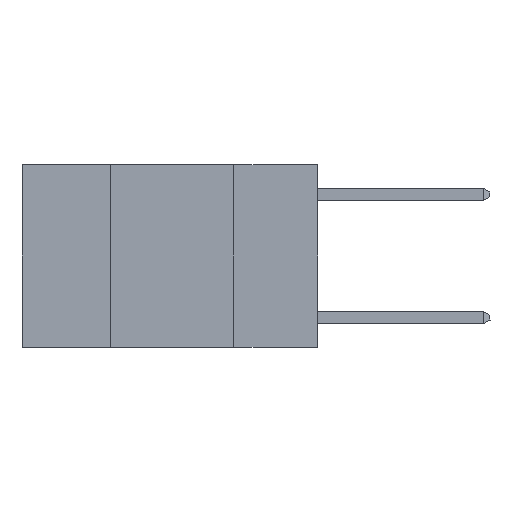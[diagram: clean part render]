
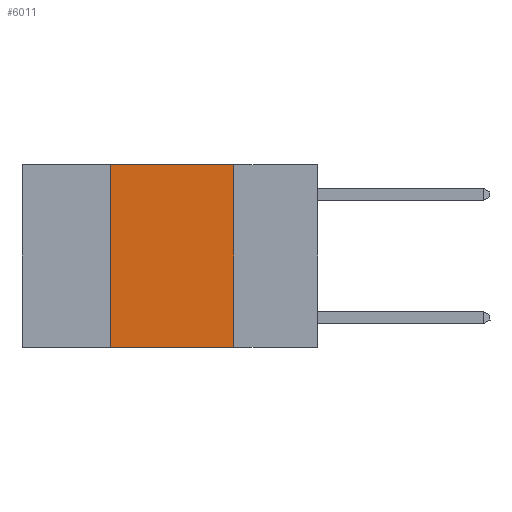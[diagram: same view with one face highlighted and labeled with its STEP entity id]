
A CAD part, left-side view. The second image highlights one B-rep face of the part: STEP entity #6011.
In plain terms, the highlighted planar face has unit normal (-1, 0, 0).
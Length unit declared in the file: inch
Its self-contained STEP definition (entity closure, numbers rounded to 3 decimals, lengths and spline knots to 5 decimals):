
#109 = DIRECTION ( 'NONE',  ( 0., 0., 1. ) ) ;
#329 = PLANE ( 'NONE',  #5812 ) ;
#442 = EDGE_CURVE ( 'NONE', #3343, #728, #18979, .T. ) ;
#728 = VERTEX_POINT ( 'NONE', #13109 ) ;
#1033 = FACE_OUTER_BOUND ( 'NONE', #8221, .T. ) ;
#1705 = ORIENTED_EDGE ( 'NONE', *, *, #16917, .F. ) ;
#2142 = DIRECTION ( 'NONE',  ( 0., 0., -1. ) ) ;
#2422 = VECTOR ( 'NONE', #9090, 39.37008 ) ;
#2716 = DIRECTION ( 'NONE',  ( 0., 0., -1. ) ) ;
#3343 = VERTEX_POINT ( 'NONE', #12059 ) ;
#5658 = ORIENTED_EDGE ( 'NONE', *, *, #22839, .F. ) ;
#5812 = AXIS2_PLACEMENT_3D ( 'NONE', #12805, #12883, #2142 ) ;
#6011 = ADVANCED_FACE ( 'NONE', ( #1033 ), #329, .F. ) ;
#7100 = VERTEX_POINT ( 'NONE', #20920 ) ;
#8221 = EDGE_LOOP ( 'NONE', ( #12911, #5658, #1705, #12975 ) ) ;
#8414 = CARTESIAN_POINT ( 'NONE',  ( 0., 0.6, 0. ) ) ;
#8637 = LINE ( 'NONE', #21348, #22038 ) ;
#9090 = DIRECTION ( 'NONE',  ( 0., -1., 0. ) ) ;
#12059 = CARTESIAN_POINT ( 'NONE',  ( 0., 0.17, 0. ) ) ;
#12805 = CARTESIAN_POINT ( 'NONE',  ( 0., 0.6, 0. ) ) ;
#12883 = DIRECTION ( 'NONE',  ( 1., 0., 0. ) ) ;
#12911 = ORIENTED_EDGE ( 'NONE', *, *, #442, .F. ) ;
#12975 = ORIENTED_EDGE ( 'NONE', *, *, #13389, .T. ) ;
#13109 = CARTESIAN_POINT ( 'NONE',  ( 0., 0.17, -0.37 ) ) ;
#13389 = EDGE_CURVE ( 'NONE', #7100, #728, #16110, .T. ) ;
#13451 = LINE ( 'NONE', #8414, #22162 ) ;
#14016 = VERTEX_POINT ( 'NONE', #21151 ) ;
#14325 = VECTOR ( 'NONE', #2716, 39.37008 ) ;
#16110 = LINE ( 'NONE', #19610, #2422 ) ;
#16917 = EDGE_CURVE ( 'NONE', #7100, #14016, #8637, .T. ) ;
#18880 = DIRECTION ( 'NONE',  ( 0., -1., 0. ) ) ;
#18979 = LINE ( 'NONE', #19137, #14325 ) ;
#19137 = CARTESIAN_POINT ( 'NONE',  ( 0., 0.17, 0. ) ) ;
#19610 = CARTESIAN_POINT ( 'NONE',  ( 0., 0.6, -0.37 ) ) ;
#20920 = CARTESIAN_POINT ( 'NONE',  ( 0., 0.42, -0.37 ) ) ;
#21151 = CARTESIAN_POINT ( 'NONE',  ( 0., 0.42, 0. ) ) ;
#21348 = CARTESIAN_POINT ( 'NONE',  ( 0., 0.42, 0. ) ) ;
#22038 = VECTOR ( 'NONE', #109, 39.37008 ) ;
#22162 = VECTOR ( 'NONE', #18880, 39.37008 ) ;
#22839 = EDGE_CURVE ( 'NONE', #14016, #3343, #13451, .T. ) ;
